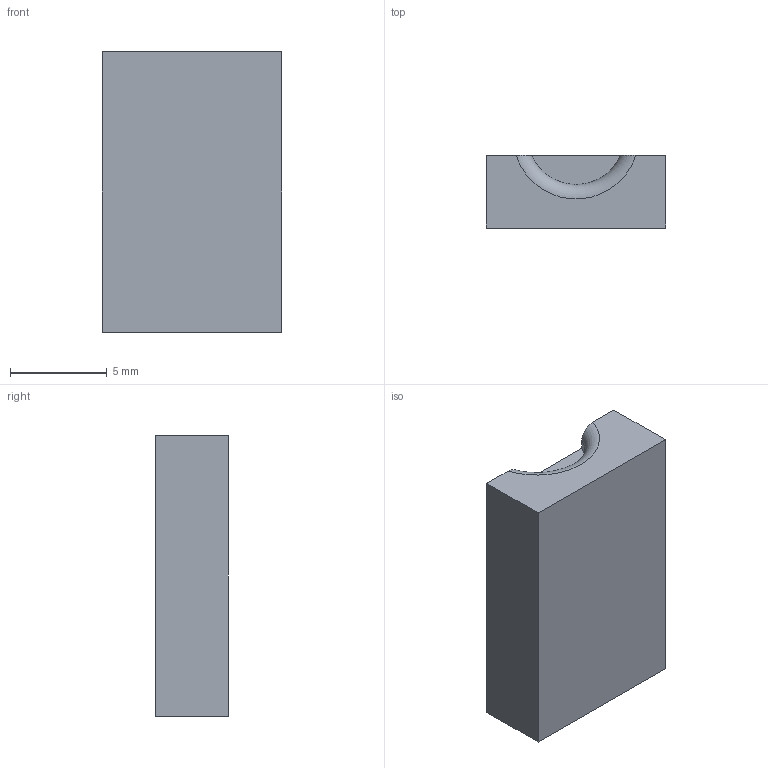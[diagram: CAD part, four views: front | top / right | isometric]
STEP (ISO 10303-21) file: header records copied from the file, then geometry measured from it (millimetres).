
FILE_DESCRIPTION (( 'STEP AP214' ), '1' );
FILE_NAME ('Thumb_Tack_Sabot.step', '2013-11-06T14:31:32', ( 'elpi' ), ( '' ), 'SwSTEP 2.0', 'SolidWorks 2013', '' );
FILE_SCHEMA (( 'AUTOMOTIVE_DESIGN' ));
Length unit declared in the file: millimetre
Products named in the file (1): Thumb_Tack_Sabot
Bounding box: 9.29 x 3.75 x 14.5 mm (x, y, z)
Volume: 400.9 mm3; surface area: 488.1 mm2
Topology: 1 solids, 1 shells, 13 faces, 33 edges, 22 vertices
Faces by surface type: plane 8, torus 3, cone 1, cylinder 1
Entity records: 488 total; most frequent: CARTESIAN_POINT 145, ORIENTED_EDGE 66, DIRECTION 60, EDGE_CURVE 33, VERTEX_POINT 22, AXIS2_PLACEMENT_3D 21, VECTOR 18, LINE 18
